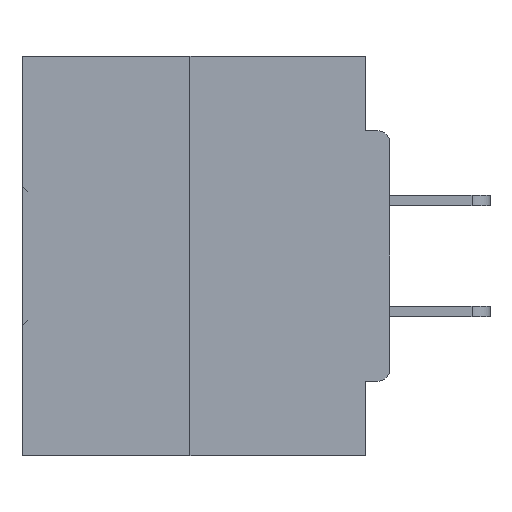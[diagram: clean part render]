
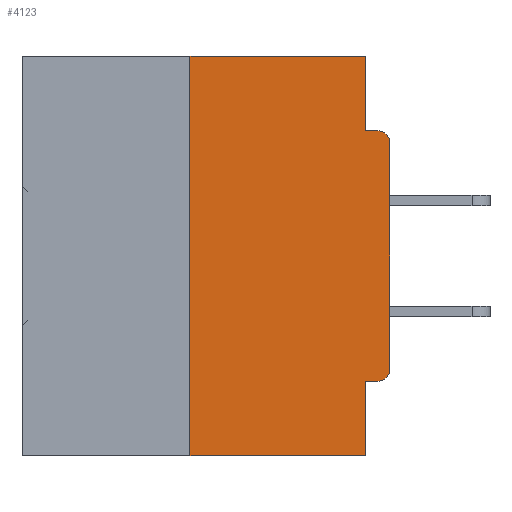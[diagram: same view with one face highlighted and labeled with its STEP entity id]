
A CAD part, left-side view. The second image highlights one B-rep face of the part: STEP entity #4123.
In plain terms, the highlighted planar face has unit normal (-1, 0, 0).
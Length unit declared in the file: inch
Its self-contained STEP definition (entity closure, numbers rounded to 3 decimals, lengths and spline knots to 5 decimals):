
#401 = AXIS2_PLACEMENT_3D ( 'NONE', #32635, #37181, #22504 ) ;
#1268 = LINE ( 'NONE', #3201, #34580 ) ;
#1397 = VECTOR ( 'NONE', #38872, 39.37008 ) ;
#1516 = EDGE_CURVE ( 'NONE', #20685, #13370, #6827, .T. ) ;
#1531 = VECTOR ( 'NONE', #2080, 39.37008 ) ;
#1713 = CARTESIAN_POINT ( 'NONE',  ( 0., 0., 0. ) ) ;
#1833 = CARTESIAN_POINT ( 'NONE',  ( 0., 0.031, -0.4065 ) ) ;
#2046 = FACE_OUTER_BOUND ( 'NONE', #17238, .T. ) ;
#2080 = DIRECTION ( 'NONE',  ( 0., 0., -1. ) ) ;
#2591 = EDGE_CURVE ( 'NONE', #7877, #34315, #19633, .T. ) ;
#2856 = CARTESIAN_POINT ( 'NONE',  ( 0., 0.031, 0. ) ) ;
#3201 = CARTESIAN_POINT ( 'NONE',  ( 0., 0., -0.4065 ) ) ;
#3491 = AXIS2_PLACEMENT_3D ( 'NONE', #41334, #34600, #26667 ) ;
#4123 = ADVANCED_FACE ( 'NONE', ( #2046 ), #21575, .F. ) ;
#4307 = CARTESIAN_POINT ( 'NONE',  ( 0., 0.25, 0. ) ) ;
#5718 = CARTESIAN_POINT ( 'NONE',  ( 0., 0.031, -0.0935 ) ) ;
#5992 = ORIENTED_EDGE ( 'NONE', *, *, #37909, .F. ) ;
#6827 = LINE ( 'NONE', #1713, #14680 ) ;
#6870 = VERTEX_POINT ( 'NONE', #14828 ) ;
#7006 = EDGE_CURVE ( 'NONE', #13370, #6870, #32234, .T. ) ;
#7877 = VERTEX_POINT ( 'NONE', #37772 ) ;
#9253 = AXIS2_PLACEMENT_3D ( 'NONE', #33182, #29835, #43728 ) ;
#9523 = VERTEX_POINT ( 'NONE', #17580 ) ;
#10167 = CARTESIAN_POINT ( 'NONE',  ( 0., 0., -0.3915 ) ) ;
#11034 = CARTESIAN_POINT ( 'NONE',  ( 0., 0.031, 0. ) ) ;
#11129 = LINE ( 'NONE', #23658, #1531 ) ;
#11480 = ORIENTED_EDGE ( 'NONE', *, *, #36157, .F. ) ;
#11507 = ORIENTED_EDGE ( 'NONE', *, *, #34769, .F. ) ;
#12159 = CARTESIAN_POINT ( 'NONE',  ( 0., 0.46, 0. ) ) ;
#13370 = VERTEX_POINT ( 'NONE', #27131 ) ;
#14680 = VECTOR ( 'NONE', #44920, 39.37008 ) ;
#14828 = CARTESIAN_POINT ( 'NONE',  ( 0., 0.015, -0.0935 ) ) ;
#15275 = EDGE_CURVE ( 'NONE', #9523, #20685, #23551, .T. ) ;
#15965 = EDGE_CURVE ( 'NONE', #30792, #19446, #33426, .T. ) ;
#16753 = VECTOR ( 'NONE', #43729, 39.37008 ) ;
#17238 = EDGE_LOOP ( 'NONE', ( #29672, #11480, #29762, #33140, #21382, #19871, #39380, #42586, #5992, #11507 ) ) ;
#17580 = CARTESIAN_POINT ( 'NONE',  ( 0., 0.015, -0.4065 ) ) ;
#18644 = VERTEX_POINT ( 'NONE', #5718 ) ;
#19041 = EDGE_CURVE ( 'NONE', #23016, #19446, #11129, .T. ) ;
#19446 = VERTEX_POINT ( 'NONE', #24995 ) ;
#19633 = LINE ( 'NONE', #12159, #23022 ) ;
#19871 = ORIENTED_EDGE ( 'NONE', *, *, #15275, .T. ) ;
#20658 = CARTESIAN_POINT ( 'NONE',  ( 0., 0., -0.0935 ) ) ;
#20685 = VERTEX_POINT ( 'NONE', #10167 ) ;
#21382 = ORIENTED_EDGE ( 'NONE', *, *, #39350, .F. ) ;
#21575 = PLANE ( 'NONE',  #401 ) ;
#22504 = DIRECTION ( 'NONE',  ( 0., 0., -1. ) ) ;
#23016 = VERTEX_POINT ( 'NONE', #1833 ) ;
#23022 = VECTOR ( 'NONE', #30790, 39.37008 ) ;
#23551 = CIRCLE ( 'NONE', #9253, 0.015 ) ;
#23658 = CARTESIAN_POINT ( 'NONE',  ( 0., 0.031, -0.5 ) ) ;
#23963 = DIRECTION ( 'NONE',  ( 0., -1., 0. ) ) ;
#24995 = CARTESIAN_POINT ( 'NONE',  ( 0., 0.031, -0.5 ) ) ;
#26667 = DIRECTION ( 'NONE',  ( 0., 0., -1. ) ) ;
#27131 = CARTESIAN_POINT ( 'NONE',  ( 0., 0., -0.1085 ) ) ;
#27217 = CARTESIAN_POINT ( 'NONE',  ( 0., 0.25, -0.5 ) ) ;
#29672 = ORIENTED_EDGE ( 'NONE', *, *, #2591, .F. ) ;
#29762 = ORIENTED_EDGE ( 'NONE', *, *, #15965, .T. ) ;
#29835 = DIRECTION ( 'NONE',  ( -1., 0., 0. ) ) ;
#30790 = DIRECTION ( 'NONE',  ( 0., -1., 0. ) ) ;
#30792 = VERTEX_POINT ( 'NONE', #27217 ) ;
#31921 = LINE ( 'NONE', #2856, #1397 ) ;
#32234 = CIRCLE ( 'NONE', #3491, 0.015 ) ;
#32384 = DIRECTION ( 'NONE',  ( 0., 1., 0. ) ) ;
#32635 = CARTESIAN_POINT ( 'NONE',  ( 0., 0.46, 0. ) ) ;
#33140 = ORIENTED_EDGE ( 'NONE', *, *, #19041, .F. ) ;
#33182 = CARTESIAN_POINT ( 'NONE',  ( 0., 0.015, -0.3915 ) ) ;
#33426 = LINE ( 'NONE', #44628, #43575 ) ;
#34315 = VERTEX_POINT ( 'NONE', #11034 ) ;
#34580 = VECTOR ( 'NONE', #32384, 39.37008 ) ;
#34600 = DIRECTION ( 'NONE',  ( -1., 0., 0. ) ) ;
#34769 = EDGE_CURVE ( 'NONE', #34315, #18644, #31921, .T. ) ;
#36157 = EDGE_CURVE ( 'NONE', #30792, #7877, #45519, .T. ) ;
#37181 = DIRECTION ( 'NONE',  ( 1., 0., 0. ) ) ;
#37529 = VECTOR ( 'NONE', #23963, 39.37008 ) ;
#37772 = CARTESIAN_POINT ( 'NONE',  ( 0., 0.25, 0. ) ) ;
#37909 = EDGE_CURVE ( 'NONE', #18644, #6870, #44849, .T. ) ;
#38872 = DIRECTION ( 'NONE',  ( 0., 0., -1. ) ) ;
#39350 = EDGE_CURVE ( 'NONE', #9523, #23016, #1268, .T. ) ;
#39380 = ORIENTED_EDGE ( 'NONE', *, *, #1516, .T. ) ;
#41006 = DIRECTION ( 'NONE',  ( 0., -1., 0. ) ) ;
#41334 = CARTESIAN_POINT ( 'NONE',  ( 0., 0.015, -0.1085 ) ) ;
#42586 = ORIENTED_EDGE ( 'NONE', *, *, #7006, .T. ) ;
#43575 = VECTOR ( 'NONE', #41006, 39.37008 ) ;
#43728 = DIRECTION ( 'NONE',  ( 0., 0., -1. ) ) ;
#43729 = DIRECTION ( 'NONE',  ( 0., 0., 1. ) ) ;
#44628 = CARTESIAN_POINT ( 'NONE',  ( 0., 0.46, -0.5 ) ) ;
#44849 = LINE ( 'NONE', #20658, #37529 ) ;
#44920 = DIRECTION ( 'NONE',  ( 0., 0., 1. ) ) ;
#45519 = LINE ( 'NONE', #4307, #16753 ) ;
